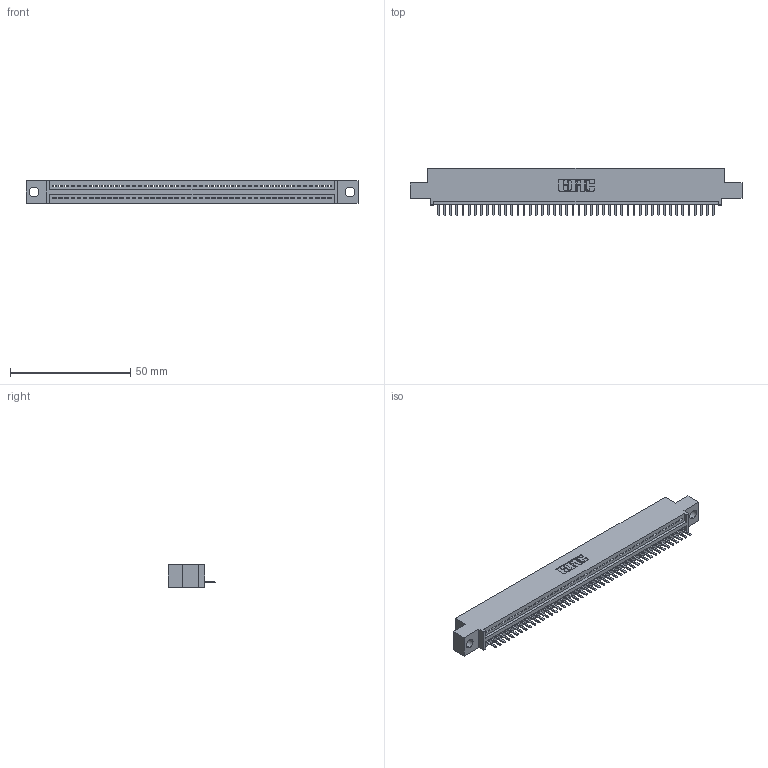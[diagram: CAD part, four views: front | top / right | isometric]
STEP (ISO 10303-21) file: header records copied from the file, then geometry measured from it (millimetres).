
FILE_DESCRIPTION (( 'STEP AP203' ), '1' );
FILE_NAME ('395-046-520-404.STEP', '2018-11-16T02:11:17', ( '' ), ( '' ), 'SwSTEP 2.0', 'SolidWorks 2016', '' );
FILE_SCHEMA (( 'CONFIG_CONTROL_DESIGN' ));
Length unit declared in the file: inch
Products named in the file (3): 395-046-520-404; 345 Part_0.110 Offset - 0.156 Dia-TH; 345-292-001_345-293-120
Assembly tree (47 placements, depth 2):
  395-046-520-404
    345 Part_0.110 Offset - 0.156 Dia-TH
    345-292-001_345-293-120  x46
Bounding box: 138.05 x 19.68 x 9.4 mm (x, y, z)
Volume: 12851.3 mm3; surface area: 16590.3 mm2
Topology: 47 solids, 47 shells, 2982 faces, 8817 edges, 5754 vertices
Faces by surface type: plane 2016, cylinder 966
Entity records: 34331 total; most frequent: CARTESIAN_POINT 5966, ORIENTED_EDGE 5934, DIRECTION 5191, EDGE_CURVE 2967, LINE 2647, VECTOR 2647, VERTEX_POINT 1974, AXIS2_PLACEMENT_3D 1272
